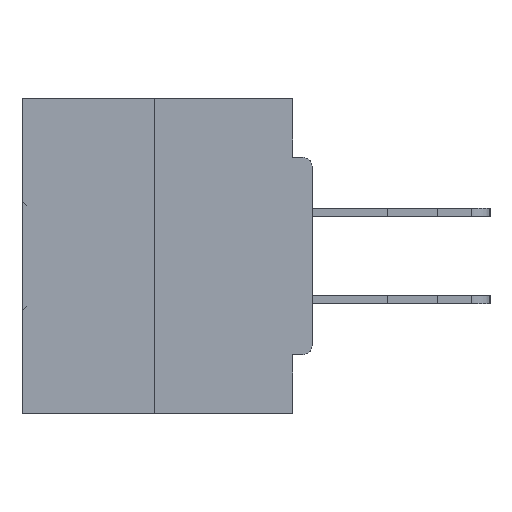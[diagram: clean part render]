
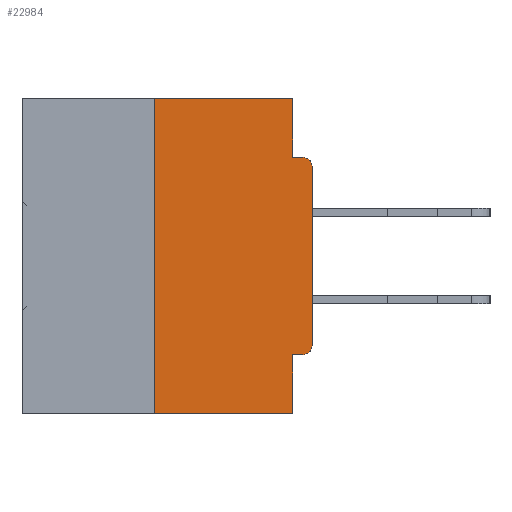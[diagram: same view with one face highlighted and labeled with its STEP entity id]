
A CAD part, left-side view. The second image highlights one B-rep face of the part: STEP entity #22984.
In plain terms, the highlighted planar face has unit normal (-1, 0, 0).
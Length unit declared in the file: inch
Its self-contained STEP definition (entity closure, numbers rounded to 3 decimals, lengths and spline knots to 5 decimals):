
#217 = EDGE_CURVE ( 'NONE', #36096, #43122, #22244, .T. ) ;
#1196 = CARTESIAN_POINT ( 'NONE',  ( 0., 0., -0.3915 ) ) ;
#2010 = DIRECTION ( 'NONE',  ( 0., 0., -1. ) ) ;
#2303 = CARTESIAN_POINT ( 'NONE',  ( 0., 0.25, 0. ) ) ;
#3639 = ORIENTED_EDGE ( 'NONE', *, *, #17010, .F. ) ;
#3675 = ORIENTED_EDGE ( 'NONE', *, *, #21703, .F. ) ;
#3887 = LINE ( 'NONE', #6397, #15405 ) ;
#4054 = EDGE_LOOP ( 'NONE', ( #27098, #3675, #6120, #38492, #45267, #28029, #4745, #12584, #3639, #9005 ) ) ;
#4745 = ORIENTED_EDGE ( 'NONE', *, *, #19961, .T. ) ;
#5722 = CARTESIAN_POINT ( 'NONE',  ( 0., 0.031, 0. ) ) ;
#5893 = DIRECTION ( 'NONE',  ( 0., 0., -1. ) ) ;
#6120 = ORIENTED_EDGE ( 'NONE', *, *, #41785, .T. ) ;
#6288 = CARTESIAN_POINT ( 'NONE',  ( 0., 0., 0. ) ) ;
#6397 = CARTESIAN_POINT ( 'NONE',  ( 0., 0.46, 0. ) ) ;
#7229 = DIRECTION ( 'NONE',  ( 0., 0., -1. ) ) ;
#7579 = CIRCLE ( 'NONE', #37102, 0.015 ) ;
#9005 = ORIENTED_EDGE ( 'NONE', *, *, #25471, .F. ) ;
#9163 = VERTEX_POINT ( 'NONE', #13218 ) ;
#11392 = CARTESIAN_POINT ( 'NONE',  ( 0., 0.031, -0.5 ) ) ;
#11440 = DIRECTION ( 'NONE',  ( -1., 0., 0. ) ) ;
#11572 = EDGE_CURVE ( 'NONE', #43122, #27315, #25740, .T. ) ;
#12584 = ORIENTED_EDGE ( 'NONE', *, *, #19345, .T. ) ;
#13218 = CARTESIAN_POINT ( 'NONE',  ( 0., 0.25, 0. ) ) ;
#13240 = VERTEX_POINT ( 'NONE', #37622 ) ;
#13546 = VECTOR ( 'NONE', #19113, 39.37008 ) ;
#13779 = DIRECTION ( 'NONE',  ( 0., -1., 0. ) ) ;
#13990 = VERTEX_POINT ( 'NONE', #45416 ) ;
#15405 = VECTOR ( 'NONE', #41505, 39.37008 ) ;
#17010 = EDGE_CURVE ( 'NONE', #13990, #13240, #36901, .T. ) ;
#17072 = VECTOR ( 'NONE', #13779, 39.37008 ) ;
#17260 = VECTOR ( 'NONE', #32397, 39.37008 ) ;
#17511 = CARTESIAN_POINT ( 'NONE',  ( 0., 0.031, -0.4065 ) ) ;
#17666 = DIRECTION ( 'NONE',  ( 0., 0., -1. ) ) ;
#17789 = EDGE_CURVE ( 'NONE', #36096, #37665, #29650, .T. ) ;
#18104 = CARTESIAN_POINT ( 'NONE',  ( 0., 0.46, -0.5 ) ) ;
#19113 = DIRECTION ( 'NONE',  ( 0., 0., 1. ) ) ;
#19188 = VECTOR ( 'NONE', #17666, 39.37008 ) ;
#19345 = EDGE_CURVE ( 'NONE', #31576, #13240, #7579, .T. ) ;
#19961 = EDGE_CURVE ( 'NONE', #37665, #31576, #33978, .T. ) ;
#20501 = DIRECTION ( 'NONE',  ( 0., 0., 1. ) ) ;
#21703 = EDGE_CURVE ( 'NONE', #29815, #9163, #32173, .T. ) ;
#22208 = DIRECTION ( 'NONE',  ( 0., 1., 0. ) ) ;
#22244 = LINE ( 'NONE', #43230, #40356 ) ;
#22984 = ADVANCED_FACE ( 'NONE', ( #38132 ), #44275, .F. ) ;
#23033 = DIRECTION ( 'NONE',  ( -1., 0., 0. ) ) ;
#23681 = CARTESIAN_POINT ( 'NONE',  ( 0., 0.46, 0. ) ) ;
#25239 = CARTESIAN_POINT ( 'NONE',  ( 0., 0.015, -0.3915 ) ) ;
#25292 = EDGE_CURVE ( 'NONE', #9163, #40424, #3887, .T. ) ;
#25471 = EDGE_CURVE ( 'NONE', #40424, #13990, #37928, .T. ) ;
#25740 = LINE ( 'NONE', #41741, #41073 ) ;
#25782 = CARTESIAN_POINT ( 'NONE',  ( 0., 0., -0.1085 ) ) ;
#26398 = CARTESIAN_POINT ( 'NONE',  ( 0., 0.25, -0.5 ) ) ;
#26915 = DIRECTION ( 'NONE',  ( 1., 0., 0. ) ) ;
#27098 = ORIENTED_EDGE ( 'NONE', *, *, #25292, .F. ) ;
#27315 = VERTEX_POINT ( 'NONE', #11392 ) ;
#28029 = ORIENTED_EDGE ( 'NONE', *, *, #17789, .T. ) ;
#29650 = CIRCLE ( 'NONE', #44441, 0.015 ) ;
#29815 = VERTEX_POINT ( 'NONE', #26398 ) ;
#31576 = VERTEX_POINT ( 'NONE', #25782 ) ;
#32173 = LINE ( 'NONE', #2303, #13546 ) ;
#32397 = DIRECTION ( 'NONE',  ( 0., -1., 0. ) ) ;
#32703 = DIRECTION ( 'NONE',  ( 0., 0., -1. ) ) ;
#33978 = LINE ( 'NONE', #6288, #36210 ) ;
#34158 = CARTESIAN_POINT ( 'NONE',  ( 0., 0., -0.0935 ) ) ;
#35696 = CARTESIAN_POINT ( 'NONE',  ( 0., 0.015, -0.4065 ) ) ;
#36096 = VERTEX_POINT ( 'NONE', #35696 ) ;
#36210 = VECTOR ( 'NONE', #20501, 39.37008 ) ;
#36556 = CARTESIAN_POINT ( 'NONE',  ( 0., 0.015, -0.1085 ) ) ;
#36644 = AXIS2_PLACEMENT_3D ( 'NONE', #23681, #26915, #5893 ) ;
#36901 = LINE ( 'NONE', #34158, #17072 ) ;
#37102 = AXIS2_PLACEMENT_3D ( 'NONE', #36556, #23033, #2010 ) ;
#37622 = CARTESIAN_POINT ( 'NONE',  ( 0., 0.015, -0.0935 ) ) ;
#37665 = VERTEX_POINT ( 'NONE', #1196 ) ;
#37928 = LINE ( 'NONE', #38752, #19188 ) ;
#38132 = FACE_OUTER_BOUND ( 'NONE', #4054, .T. ) ;
#38492 = ORIENTED_EDGE ( 'NONE', *, *, #11572, .F. ) ;
#38752 = CARTESIAN_POINT ( 'NONE',  ( 0., 0.031, 0. ) ) ;
#40356 = VECTOR ( 'NONE', #22208, 39.37008 ) ;
#40424 = VERTEX_POINT ( 'NONE', #5722 ) ;
#41073 = VECTOR ( 'NONE', #7229, 39.37008 ) ;
#41427 = LINE ( 'NONE', #18104, #17260 ) ;
#41505 = DIRECTION ( 'NONE',  ( 0., -1., 0. ) ) ;
#41741 = CARTESIAN_POINT ( 'NONE',  ( 0., 0.031, -0.5 ) ) ;
#41785 = EDGE_CURVE ( 'NONE', #29815, #27315, #41427, .T. ) ;
#43122 = VERTEX_POINT ( 'NONE', #17511 ) ;
#43230 = CARTESIAN_POINT ( 'NONE',  ( 0., 0., -0.4065 ) ) ;
#44275 = PLANE ( 'NONE',  #36644 ) ;
#44441 = AXIS2_PLACEMENT_3D ( 'NONE', #25239, #11440, #32703 ) ;
#45267 = ORIENTED_EDGE ( 'NONE', *, *, #217, .F. ) ;
#45416 = CARTESIAN_POINT ( 'NONE',  ( 0., 0.031, -0.0935 ) ) ;
